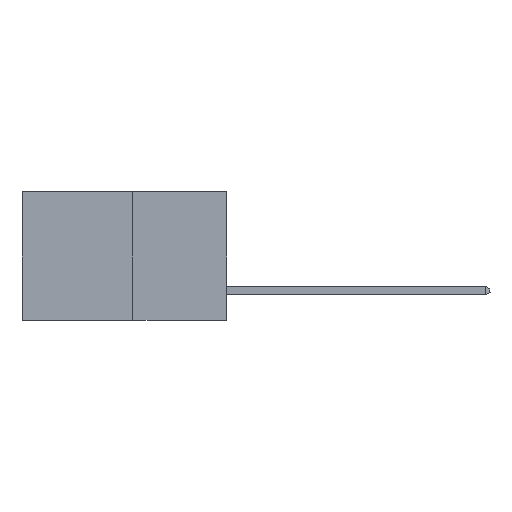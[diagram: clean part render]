
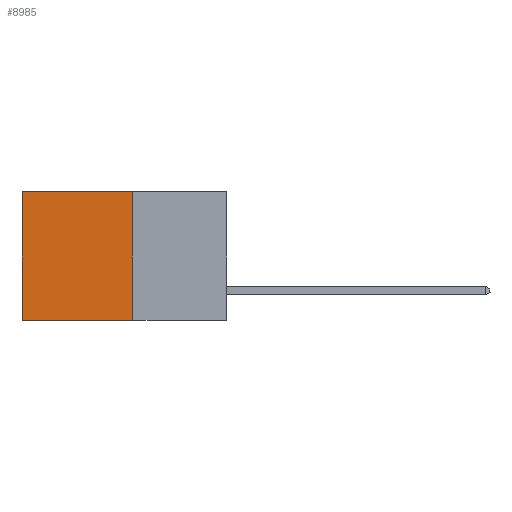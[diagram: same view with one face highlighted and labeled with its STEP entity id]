
A CAD part, left-side view. The second image highlights one B-rep face of the part: STEP entity #8985.
In plain terms, the highlighted planar face has unit normal (-1, 0, 0).
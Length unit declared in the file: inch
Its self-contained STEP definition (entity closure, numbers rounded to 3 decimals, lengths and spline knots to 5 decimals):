
#498 = EDGE_CURVE ( 'NONE', #12257, #2993, #5292, .T. ) ;
#798 = CARTESIAN_POINT ( 'NONE',  ( 0.277, 0.27, -0.37 ) ) ;
#1467 = EDGE_CURVE ( 'NONE', #12087, #12257, #12595, .T. ) ;
#1642 = CARTESIAN_POINT ( 'NONE',  ( 0.277, 0.59, -0.37 ) ) ;
#1721 = VERTEX_POINT ( 'NONE', #12533 ) ;
#1958 = FACE_OUTER_BOUND ( 'NONE', #10299, .T. ) ;
#2391 = CARTESIAN_POINT ( 'NONE',  ( 0.277, 0.27, -0.37 ) ) ;
#2859 = DIRECTION ( 'NONE',  ( 0., 0., -1. ) ) ;
#2993 = VERTEX_POINT ( 'NONE', #10611 ) ;
#3496 = DIRECTION ( 'NONE',  ( 0., 0., -1. ) ) ;
#3507 = VECTOR ( 'NONE', #3496, 39.37008 ) ;
#4066 = DIRECTION ( 'NONE',  ( 1., 0., 0. ) ) ;
#5292 = LINE ( 'NONE', #1642, #10531 ) ;
#5426 = EDGE_CURVE ( 'NONE', #1721, #2993, #8285, .T. ) ;
#5804 = VECTOR ( 'NONE', #10739, 39.37008 ) ;
#6115 = AXIS2_PLACEMENT_3D ( 'NONE', #798, #4066, #11384 ) ;
#6311 = LINE ( 'NONE', #2391, #3507 ) ;
#7993 = ORIENTED_EDGE ( 'NONE', *, *, #5426, .F. ) ;
#8237 = EDGE_CURVE ( 'NONE', #12087, #1721, #6311, .T. ) ;
#8285 = LINE ( 'NONE', #11775, #5804 ) ;
#8978 = ORIENTED_EDGE ( 'NONE', *, *, #1467, .T. ) ;
#8985 = ADVANCED_FACE ( 'NONE', ( #1958 ), #13327, .F. ) ;
#10299 = EDGE_LOOP ( 'NONE', ( #13129, #7993, #11719, #8978 ) ) ;
#10425 = CARTESIAN_POINT ( 'NONE',  ( 0.277, 0.59, 0. ) ) ;
#10526 = DIRECTION ( 'NONE',  ( 0., 1., 0. ) ) ;
#10531 = VECTOR ( 'NONE', #2859, 39.37008 ) ;
#10611 = CARTESIAN_POINT ( 'NONE',  ( 0.277, 0.59, -0.37 ) ) ;
#10625 = CARTESIAN_POINT ( 'NONE',  ( 0.277, 0.27, 0. ) ) ;
#10739 = DIRECTION ( 'NONE',  ( 0., 1., 0. ) ) ;
#11384 = DIRECTION ( 'NONE',  ( 0., 0., -1. ) ) ;
#11719 = ORIENTED_EDGE ( 'NONE', *, *, #8237, .F. ) ;
#11775 = CARTESIAN_POINT ( 'NONE',  ( 0.277, 0.27, -0.37 ) ) ;
#12087 = VERTEX_POINT ( 'NONE', #13186 ) ;
#12257 = VERTEX_POINT ( 'NONE', #10425 ) ;
#12533 = CARTESIAN_POINT ( 'NONE',  ( 0.277, 0.27, -0.37 ) ) ;
#12595 = LINE ( 'NONE', #10625, #12908 ) ;
#12908 = VECTOR ( 'NONE', #10526, 39.37008 ) ;
#13129 = ORIENTED_EDGE ( 'NONE', *, *, #498, .T. ) ;
#13186 = CARTESIAN_POINT ( 'NONE',  ( 0.277, 0.27, 0. ) ) ;
#13327 = PLANE ( 'NONE',  #6115 ) ;
